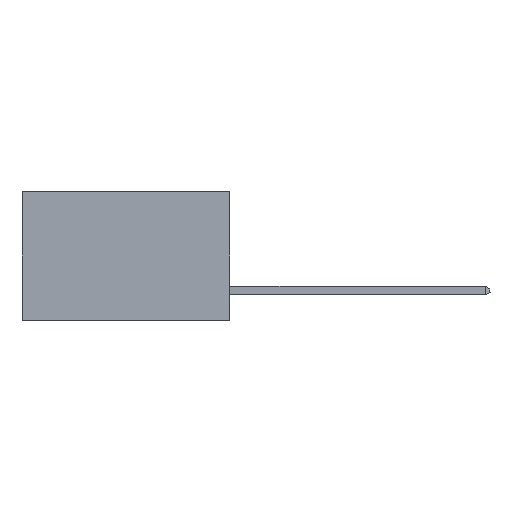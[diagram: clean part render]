
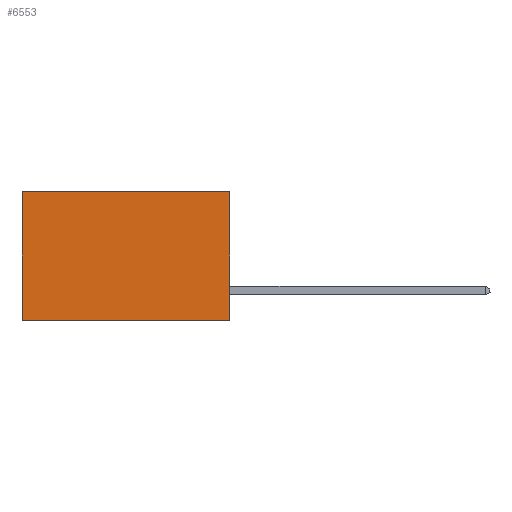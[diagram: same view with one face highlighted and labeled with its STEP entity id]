
A CAD part, left-side view. The second image highlights one B-rep face of the part: STEP entity #6553.
In plain terms, the highlighted planar face has unit normal (-1, 0, 0).
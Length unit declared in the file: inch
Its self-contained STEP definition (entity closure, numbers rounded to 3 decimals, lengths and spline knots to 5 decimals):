
#1525 = VECTOR ( 'NONE', #13316, 39.37008 ) ;
#2940 = VECTOR ( 'NONE', #3365, 39.37008 ) ;
#3365 = DIRECTION ( 'NONE',  ( 0., 1., 0. ) ) ;
#4339 = DIRECTION ( 'NONE',  ( 1., 0., 0. ) ) ;
#5153 = DIRECTION ( 'NONE',  ( 0., 0., -1. ) ) ;
#5215 = VERTEX_POINT ( 'NONE', #28651 ) ;
#6106 = CARTESIAN_POINT ( 'NONE',  ( 0.298, 0., 0. ) ) ;
#6553 = ADVANCED_FACE ( 'NONE', ( #14631 ), #9079, .F. ) ;
#6564 = CARTESIAN_POINT ( 'NONE',  ( 0.298, 0., 0. ) ) ;
#9079 = PLANE ( 'NONE',  #27614 ) ;
#9116 = EDGE_LOOP ( 'NONE', ( #12454, #25612, #15452, #14534 ) ) ;
#9455 = LINE ( 'NONE', #6106, #1525 ) ;
#10579 = LINE ( 'NONE', #14479, #16309 ) ;
#11075 = CARTESIAN_POINT ( 'NONE',  ( 0.298, 0.6, 0. ) ) ;
#12424 = LINE ( 'NONE', #6564, #24579 ) ;
#12454 = ORIENTED_EDGE ( 'NONE', *, *, #31226, .T. ) ;
#13316 = DIRECTION ( 'NONE',  ( 0., 0., -1. ) ) ;
#14479 = CARTESIAN_POINT ( 'NONE',  ( 0.298, 0.6, 0. ) ) ;
#14534 = ORIENTED_EDGE ( 'NONE', *, *, #17391, .T. ) ;
#14631 = FACE_OUTER_BOUND ( 'NONE', #9116, .T. ) ;
#15452 = ORIENTED_EDGE ( 'NONE', *, *, #30837, .F. ) ;
#15644 = VERTEX_POINT ( 'NONE', #11075 ) ;
#15819 = LINE ( 'NONE', #25007, #2940 ) ;
#15873 = VERTEX_POINT ( 'NONE', #28526 ) ;
#16309 = VECTOR ( 'NONE', #5153, 39.37008 ) ;
#17391 = EDGE_CURVE ( 'NONE', #5215, #15644, #12424, .T. ) ;
#18645 = DIRECTION ( 'NONE',  ( 0., 1., 0. ) ) ;
#21268 = DIRECTION ( 'NONE',  ( 0., 0., -1. ) ) ;
#22830 = EDGE_CURVE ( 'NONE', #24941, #15873, #15819, .T. ) ;
#22871 = CARTESIAN_POINT ( 'NONE',  ( 0.298, 0., -0.37 ) ) ;
#24579 = VECTOR ( 'NONE', #18645, 39.37008 ) ;
#24941 = VERTEX_POINT ( 'NONE', #22871 ) ;
#25007 = CARTESIAN_POINT ( 'NONE',  ( 0.298, 0., -0.37 ) ) ;
#25612 = ORIENTED_EDGE ( 'NONE', *, *, #22830, .F. ) ;
#27614 = AXIS2_PLACEMENT_3D ( 'NONE', #30940, #4339, #21268 ) ;
#28526 = CARTESIAN_POINT ( 'NONE',  ( 0.298, 0.6, -0.37 ) ) ;
#28651 = CARTESIAN_POINT ( 'NONE',  ( 0.298, 0., 0. ) ) ;
#30837 = EDGE_CURVE ( 'NONE', #5215, #24941, #9455, .T. ) ;
#30940 = CARTESIAN_POINT ( 'NONE',  ( 0.298, 0., 0. ) ) ;
#31226 = EDGE_CURVE ( 'NONE', #15644, #15873, #10579, .T. ) ;
